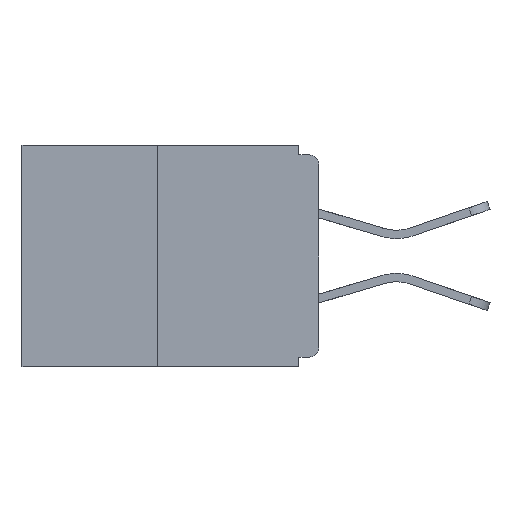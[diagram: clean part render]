
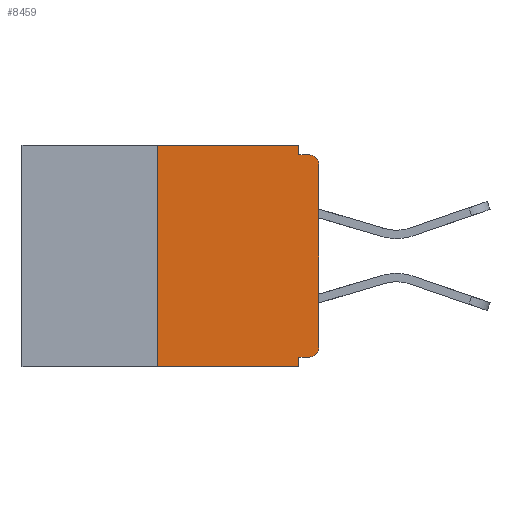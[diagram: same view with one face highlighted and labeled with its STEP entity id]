
A CAD part, left-side view. The second image highlights one B-rep face of the part: STEP entity #8459.
In plain terms, the highlighted planar face has unit normal (-1, 0, 0).
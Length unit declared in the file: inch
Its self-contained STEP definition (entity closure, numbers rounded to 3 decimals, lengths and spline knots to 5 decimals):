
#289 = ORIENTED_EDGE ( 'NONE', *, *, #9785, .T. ) ;
#290 = ORIENTED_EDGE ( 'NONE', *, *, #11519, .F. ) ;
#297 = ORIENTED_EDGE ( 'NONE', *, *, #7422, .F. ) ;
#310 = CARTESIAN_POINT ( 'NONE',  ( 0., 0.015, -0.328 ) ) ;
#355 = CARTESIAN_POINT ( 'NONE',  ( 0., 0.031, -0.015 ) ) ;
#377 = AXIS2_PLACEMENT_3D ( 'NONE', #1604, #11245, #2622 ) ;
#469 = VECTOR ( 'NONE', #10601, 39.37008 ) ;
#532 = VERTEX_POINT ( 'NONE', #355 ) ;
#582 = LINE ( 'NONE', #2387, #10580 ) ;
#843 = LINE ( 'NONE', #1891, #2978 ) ;
#848 = VERTEX_POINT ( 'NONE', #8668 ) ;
#1347 = VERTEX_POINT ( 'NONE', #4387 ) ;
#1543 = DIRECTION ( 'NONE',  ( 0., 0., 1. ) ) ;
#1604 = CARTESIAN_POINT ( 'NONE',  ( 0., 0.015, -0.313 ) ) ;
#1871 = CARTESIAN_POINT ( 'NONE',  ( 0., 0.031, -0.343 ) ) ;
#1891 = CARTESIAN_POINT ( 'NONE',  ( 0., 0.031, -0.343 ) ) ;
#1915 = CARTESIAN_POINT ( 'NONE',  ( 0., 0.031, -0.328 ) ) ;
#2096 = ORIENTED_EDGE ( 'NONE', *, *, #10244, .F. ) ;
#2387 = CARTESIAN_POINT ( 'NONE',  ( 0., 0.25, 0. ) ) ;
#2391 = EDGE_CURVE ( 'NONE', #3731, #6477, #4729, .T. ) ;
#2532 = VECTOR ( 'NONE', #8813, 39.37008 ) ;
#2622 = DIRECTION ( 'NONE',  ( 0., 0., -1. ) ) ;
#2757 = DIRECTION ( 'NONE',  ( 0., 0., 1. ) ) ;
#2978 = VECTOR ( 'NONE', #4833, 39.37008 ) ;
#3091 = VECTOR ( 'NONE', #11032, 39.37008 ) ;
#3250 = DIRECTION ( 'NONE',  ( 1., 0., 0. ) ) ;
#3270 = ORIENTED_EDGE ( 'NONE', *, *, #4961, .F. ) ;
#3363 = DIRECTION ( 'NONE',  ( -1., 0., 0. ) ) ;
#3571 = ORIENTED_EDGE ( 'NONE', *, *, #4413, .F. ) ;
#3731 = VERTEX_POINT ( 'NONE', #4000 ) ;
#3845 = CARTESIAN_POINT ( 'NONE',  ( 0., 0.46, 0. ) ) ;
#4000 = CARTESIAN_POINT ( 'NONE',  ( 0., 0.25, -0.343 ) ) ;
#4004 = AXIS2_PLACEMENT_3D ( 'NONE', #4241, #3250, #10972 ) ;
#4241 = CARTESIAN_POINT ( 'NONE',  ( 0., 0.46, 0. ) ) ;
#4245 = EDGE_CURVE ( 'NONE', #11438, #848, #5851, .T. ) ;
#4377 = VERTEX_POINT ( 'NONE', #310 ) ;
#4387 = CARTESIAN_POINT ( 'NONE',  ( 0., 0.25, 0. ) ) ;
#4413 = EDGE_CURVE ( 'NONE', #532, #10286, #5210, .T. ) ;
#4729 = LINE ( 'NONE', #5798, #12101 ) ;
#4833 = DIRECTION ( 'NONE',  ( 0., 0., -1. ) ) ;
#4961 = EDGE_CURVE ( 'NONE', #1347, #5793, #5339, .T. ) ;
#5056 = EDGE_CURVE ( 'NONE', #4377, #11438, #12248, .T. ) ;
#5125 = ORIENTED_EDGE ( 'NONE', *, *, #2391, .T. ) ;
#5210 = LINE ( 'NONE', #8072, #3091 ) ;
#5218 = VECTOR ( 'NONE', #2757, 39.37008 ) ;
#5339 = LINE ( 'NONE', #3845, #469 ) ;
#5615 = CARTESIAN_POINT ( 'NONE',  ( 0., 0.031, 0. ) ) ;
#5652 = AXIS2_PLACEMENT_3D ( 'NONE', #12042, #3363, #6336 ) ;
#5793 = VERTEX_POINT ( 'NONE', #10389 ) ;
#5798 = CARTESIAN_POINT ( 'NONE',  ( 0., 0.46, -0.343 ) ) ;
#5851 = LINE ( 'NONE', #11457, #5218 ) ;
#6069 = LINE ( 'NONE', #5615, #11897 ) ;
#6336 = DIRECTION ( 'NONE',  ( 0., 0., -1. ) ) ;
#6477 = VERTEX_POINT ( 'NONE', #1871 ) ;
#6962 = EDGE_LOOP ( 'NONE', ( #3270, #297, #5125, #12098, #290, #10394, #7670, #289, #3571, #2096 ) ) ;
#7371 = CARTESIAN_POINT ( 'NONE',  ( 0., 0.015, -0.015 ) ) ;
#7422 = EDGE_CURVE ( 'NONE', #3731, #1347, #582, .T. ) ;
#7640 = DIRECTION ( 'NONE',  ( 0., -1., 0. ) ) ;
#7670 = ORIENTED_EDGE ( 'NONE', *, *, #4245, .T. ) ;
#7889 = CARTESIAN_POINT ( 'NONE',  ( 0., 0., -0.328 ) ) ;
#8072 = CARTESIAN_POINT ( 'NONE',  ( 0., 0., -0.015 ) ) ;
#8278 = LINE ( 'NONE', #7889, #2532 ) ;
#8459 = ADVANCED_FACE ( 'NONE', ( #12028 ), #10019, .F. ) ;
#8638 = CARTESIAN_POINT ( 'NONE',  ( 0., 0., -0.313 ) ) ;
#8668 = CARTESIAN_POINT ( 'NONE',  ( 0., 0., -0.03 ) ) ;
#8813 = DIRECTION ( 'NONE',  ( 0., 1., 0. ) ) ;
#9785 = EDGE_CURVE ( 'NONE', #848, #10286, #12196, .T. ) ;
#10019 = PLANE ( 'NONE',  #4004 ) ;
#10244 = EDGE_CURVE ( 'NONE', #5793, #532, #6069, .T. ) ;
#10286 = VERTEX_POINT ( 'NONE', #7371 ) ;
#10360 = VERTEX_POINT ( 'NONE', #1915 ) ;
#10389 = CARTESIAN_POINT ( 'NONE',  ( 0., 0.031, 0. ) ) ;
#10394 = ORIENTED_EDGE ( 'NONE', *, *, #5056, .T. ) ;
#10580 = VECTOR ( 'NONE', #1543, 39.37008 ) ;
#10601 = DIRECTION ( 'NONE',  ( 0., -1., 0. ) ) ;
#10972 = DIRECTION ( 'NONE',  ( 0., 0., -1. ) ) ;
#11032 = DIRECTION ( 'NONE',  ( 0., -1., 0. ) ) ;
#11245 = DIRECTION ( 'NONE',  ( -1., 0., 0. ) ) ;
#11423 = EDGE_CURVE ( 'NONE', #10360, #6477, #843, .T. ) ;
#11438 = VERTEX_POINT ( 'NONE', #8638 ) ;
#11457 = CARTESIAN_POINT ( 'NONE',  ( 0., 0., 0. ) ) ;
#11519 = EDGE_CURVE ( 'NONE', #4377, #10360, #8278, .T. ) ;
#11897 = VECTOR ( 'NONE', #12202, 39.37008 ) ;
#12028 = FACE_OUTER_BOUND ( 'NONE', #6962, .T. ) ;
#12042 = CARTESIAN_POINT ( 'NONE',  ( 0., 0.015, -0.03 ) ) ;
#12098 = ORIENTED_EDGE ( 'NONE', *, *, #11423, .F. ) ;
#12101 = VECTOR ( 'NONE', #7640, 39.37008 ) ;
#12196 = CIRCLE ( 'NONE', #5652, 0.015 ) ;
#12202 = DIRECTION ( 'NONE',  ( 0., 0., -1. ) ) ;
#12248 = CIRCLE ( 'NONE', #377, 0.015 ) ;
